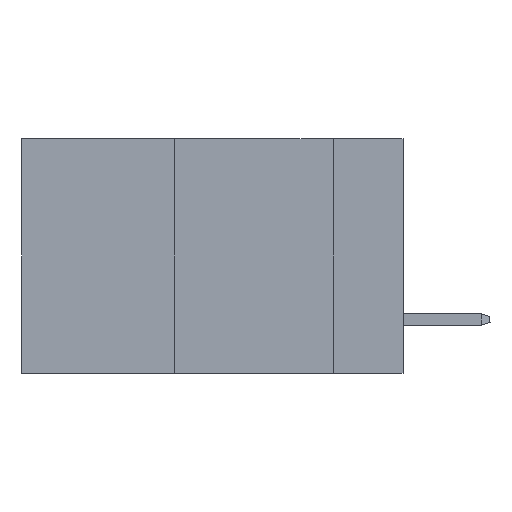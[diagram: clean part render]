
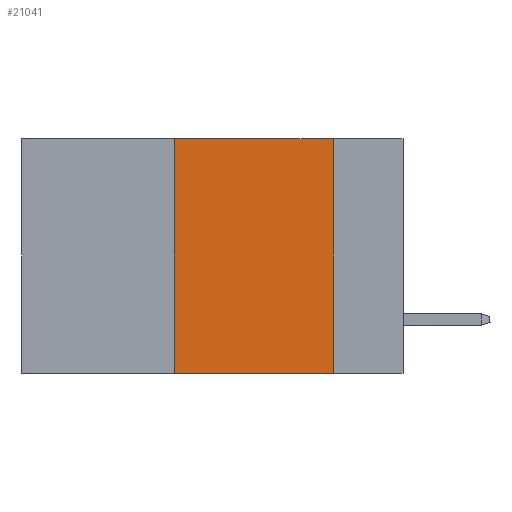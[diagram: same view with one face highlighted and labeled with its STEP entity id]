
A CAD part, left-side view. The second image highlights one B-rep face of the part: STEP entity #21041.
In plain terms, the highlighted planar face has unit normal (-1, 0, 0).
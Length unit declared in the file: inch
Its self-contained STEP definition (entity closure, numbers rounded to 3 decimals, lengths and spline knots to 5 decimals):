
#795 = FACE_OUTER_BOUND ( 'NONE', #23625, .T. ) ;
#1216 = VERTEX_POINT ( 'NONE', #5727 ) ;
#1781 = VECTOR ( 'NONE', #15987, 39.37008 ) ;
#1854 = CARTESIAN_POINT ( 'NONE',  ( 0., 0.11, 0. ) ) ;
#2425 = EDGE_CURVE ( 'NONE', #15512, #6051, #3684, .T. ) ;
#3128 = DIRECTION ( 'NONE',  ( 0., 0., -1. ) ) ;
#3684 = LINE ( 'NONE', #21795, #15504 ) ;
#4404 = ORIENTED_EDGE ( 'NONE', *, *, #9013, .F. ) ;
#4627 = DIRECTION ( 'NONE',  ( 0., -1., 0. ) ) ;
#5327 = CARTESIAN_POINT ( 'NONE',  ( 0., 0.36, 0. ) ) ;
#5727 = CARTESIAN_POINT ( 'NONE',  ( 0., 0.11, 0. ) ) ;
#6051 = VERTEX_POINT ( 'NONE', #9524 ) ;
#6984 = CARTESIAN_POINT ( 'NONE',  ( 0., 0.6, 0. ) ) ;
#6989 = EDGE_CURVE ( 'NONE', #1216, #6051, #15943, .T. ) ;
#7914 = DIRECTION ( 'NONE',  ( 0., 0., -1. ) ) ;
#8112 = CARTESIAN_POINT ( 'NONE',  ( 0., 0.6, 0. ) ) ;
#9013 = EDGE_CURVE ( 'NONE', #14353, #1216, #19884, .T. ) ;
#9524 = CARTESIAN_POINT ( 'NONE',  ( 0., 0.11, -0.37 ) ) ;
#9549 = AXIS2_PLACEMENT_3D ( 'NONE', #6984, #22673, #3128 ) ;
#10171 = CARTESIAN_POINT ( 'NONE',  ( 0., 0.36, 0. ) ) ;
#11883 = VECTOR ( 'NONE', #4627, 39.37008 ) ;
#12382 = CARTESIAN_POINT ( 'NONE',  ( 0., 0.36, -0.37 ) ) ;
#12879 = ORIENTED_EDGE ( 'NONE', *, *, #2425, .T. ) ;
#13526 = ORIENTED_EDGE ( 'NONE', *, *, #18727, .F. ) ;
#13872 = VECTOR ( 'NONE', #7914, 39.37008 ) ;
#14353 = VERTEX_POINT ( 'NONE', #5327 ) ;
#14892 = PLANE ( 'NONE',  #9549 ) ;
#15504 = VECTOR ( 'NONE', #23490, 39.37008 ) ;
#15512 = VERTEX_POINT ( 'NONE', #12382 ) ;
#15943 = LINE ( 'NONE', #1854, #13872 ) ;
#15987 = DIRECTION ( 'NONE',  ( 0., 0., 1. ) ) ;
#18727 = EDGE_CURVE ( 'NONE', #15512, #14353, #21954, .T. ) ;
#19884 = LINE ( 'NONE', #8112, #11883 ) ;
#21041 = ADVANCED_FACE ( 'NONE', ( #795 ), #14892, .F. ) ;
#21795 = CARTESIAN_POINT ( 'NONE',  ( 0., 0.6, -0.37 ) ) ;
#21954 = LINE ( 'NONE', #10171, #1781 ) ;
#22673 = DIRECTION ( 'NONE',  ( 1., 0., 0. ) ) ;
#23490 = DIRECTION ( 'NONE',  ( 0., -1., 0. ) ) ;
#23625 = EDGE_LOOP ( 'NONE', ( #24589, #4404, #13526, #12879 ) ) ;
#24589 = ORIENTED_EDGE ( 'NONE', *, *, #6989, .F. ) ;
